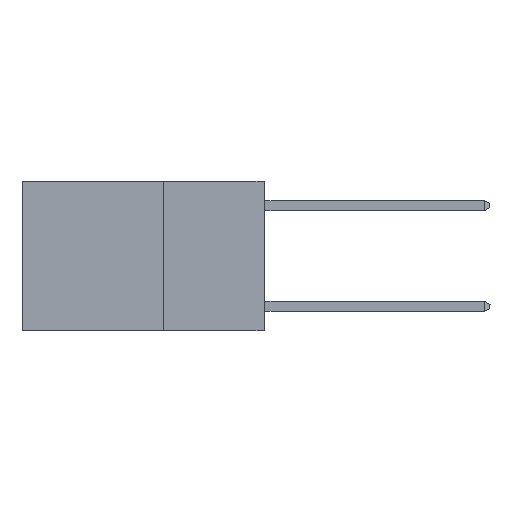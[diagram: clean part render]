
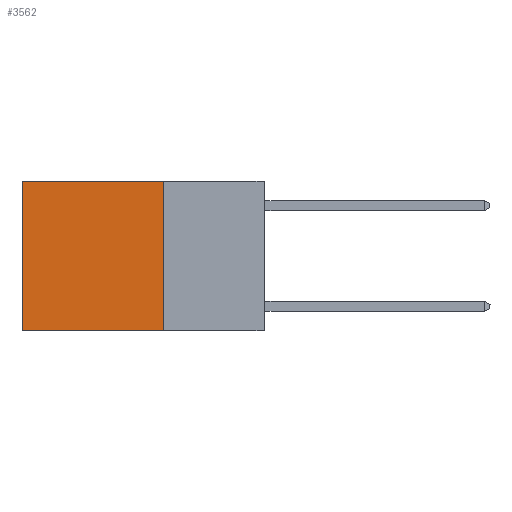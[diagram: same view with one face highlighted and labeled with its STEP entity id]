
A CAD part, left-side view. The second image highlights one B-rep face of the part: STEP entity #3562.
In plain terms, the highlighted planar face has unit normal (-1, 0, 0).
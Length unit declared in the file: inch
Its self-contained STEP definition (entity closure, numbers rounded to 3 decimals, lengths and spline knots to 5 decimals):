
#111 = DIRECTION ( 'NONE',  ( 1., 0., 0. ) ) ;
#273 = FACE_OUTER_BOUND ( 'NONE', #12374, .T. ) ;
#1207 = CARTESIAN_POINT ( 'NONE',  ( 0.2625, 0.6, 0. ) ) ;
#1579 = VERTEX_POINT ( 'NONE', #14141 ) ;
#1836 = VECTOR ( 'NONE', #5833, 39.37008 ) ;
#2366 = CARTESIAN_POINT ( 'NONE',  ( 0.2625, 0.25, -0.37 ) ) ;
#2571 = LINE ( 'NONE', #7565, #10331 ) ;
#2649 = ORIENTED_EDGE ( 'NONE', *, *, #13686, .F. ) ;
#3318 = LINE ( 'NONE', #12666, #13986 ) ;
#3562 = ADVANCED_FACE ( 'NONE', ( #273 ), #7400, .F. ) ;
#4344 = CARTESIAN_POINT ( 'NONE',  ( 0.2625, 0.25, 0. ) ) ;
#5498 = DIRECTION ( 'NONE',  ( 0., 1., 0. ) ) ;
#5833 = DIRECTION ( 'NONE',  ( 0., 0., -1. ) ) ;
#6214 = LINE ( 'NONE', #4344, #1836 ) ;
#7400 = PLANE ( 'NONE',  #15463 ) ;
#7565 = CARTESIAN_POINT ( 'NONE',  ( 0.2625, 0.25, -0.37 ) ) ;
#7828 = VERTEX_POINT ( 'NONE', #2366 ) ;
#10322 = DIRECTION ( 'NONE',  ( 0., 0., -1. ) ) ;
#10331 = VECTOR ( 'NONE', #16213, 39.37008 ) ;
#11044 = CARTESIAN_POINT ( 'NONE',  ( 0.2625, 0.6, -0.37 ) ) ;
#11593 = ORIENTED_EDGE ( 'NONE', *, *, #16967, .T. ) ;
#12374 = EDGE_LOOP ( 'NONE', ( #11593, #2649, #18730, #15937 ) ) ;
#12666 = CARTESIAN_POINT ( 'NONE',  ( 0.2625, 0.25, 0. ) ) ;
#12679 = LINE ( 'NONE', #1207, #16038 ) ;
#13686 = EDGE_CURVE ( 'NONE', #7828, #13912, #2571, .T. ) ;
#13912 = VERTEX_POINT ( 'NONE', #11044 ) ;
#13986 = VECTOR ( 'NONE', #5498, 39.37008 ) ;
#14141 = CARTESIAN_POINT ( 'NONE',  ( 0.2625, 0.25, 0. ) ) ;
#14819 = EDGE_CURVE ( 'NONE', #1579, #7828, #6214, .T. ) ;
#15463 = AXIS2_PLACEMENT_3D ( 'NONE', #17502, #111, #10322 ) ;
#15555 = CARTESIAN_POINT ( 'NONE',  ( 0.2625, 0.6, 0. ) ) ;
#15562 = VERTEX_POINT ( 'NONE', #15555 ) ;
#15760 = DIRECTION ( 'NONE',  ( 0., 0., -1. ) ) ;
#15937 = ORIENTED_EDGE ( 'NONE', *, *, #17598, .T. ) ;
#16038 = VECTOR ( 'NONE', #15760, 39.37008 ) ;
#16213 = DIRECTION ( 'NONE',  ( 0., 1., 0. ) ) ;
#16967 = EDGE_CURVE ( 'NONE', #15562, #13912, #12679, .T. ) ;
#17502 = CARTESIAN_POINT ( 'NONE',  ( 0.2625, 0.25, 0. ) ) ;
#17598 = EDGE_CURVE ( 'NONE', #1579, #15562, #3318, .T. ) ;
#18730 = ORIENTED_EDGE ( 'NONE', *, *, #14819, .F. ) ;
